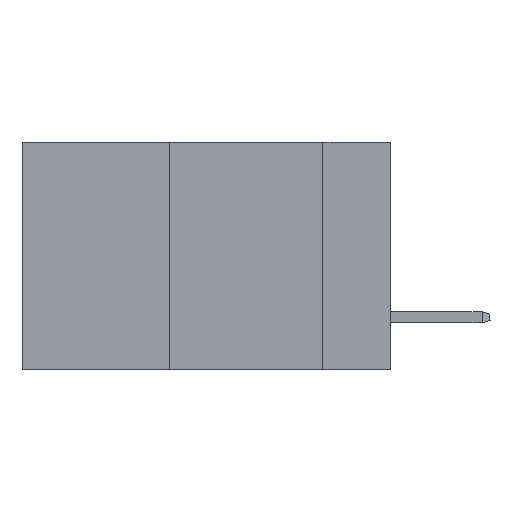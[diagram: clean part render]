
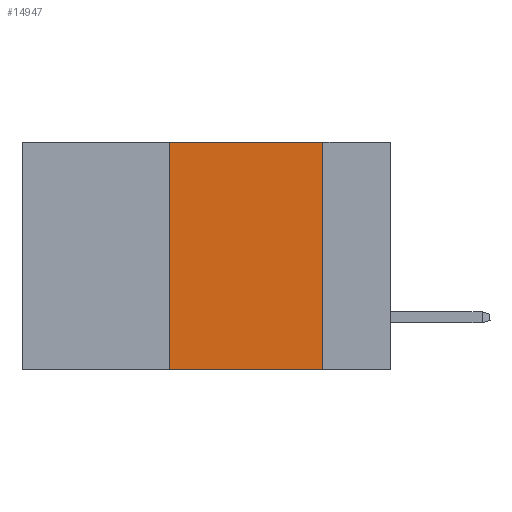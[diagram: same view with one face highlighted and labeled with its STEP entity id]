
A CAD part, left-side view. The second image highlights one B-rep face of the part: STEP entity #14947.
In plain terms, the highlighted planar face has unit normal (-1, 0, 0).
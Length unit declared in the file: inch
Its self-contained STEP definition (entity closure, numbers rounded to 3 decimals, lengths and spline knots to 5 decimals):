
#177 = VECTOR ( 'NONE', #9174, 39.37008 ) ;
#655 = VERTEX_POINT ( 'NONE', #10690 ) ;
#737 = CARTESIAN_POINT ( 'NONE',  ( 0., 0.6, 0. ) ) ;
#1632 = ORIENTED_EDGE ( 'NONE', *, *, #12199, .T. ) ;
#1851 = DIRECTION ( 'NONE',  ( 0., 0., -1. ) ) ;
#2074 = VECTOR ( 'NONE', #1851, 39.37008 ) ;
#2900 = CARTESIAN_POINT ( 'NONE',  ( 0., 0.36, 0. ) ) ;
#2974 = VECTOR ( 'NONE', #7356, 39.37008 ) ;
#4194 = LINE ( 'NONE', #6537, #2074 ) ;
#5190 = DIRECTION ( 'NONE',  ( 0., -1., 0. ) ) ;
#5197 = DIRECTION ( 'NONE',  ( 0., 0., -1. ) ) ;
#5221 = VECTOR ( 'NONE', #5190, 39.37008 ) ;
#5505 = VERTEX_POINT ( 'NONE', #14729 ) ;
#6537 = CARTESIAN_POINT ( 'NONE',  ( 0., 0.11, 0. ) ) ;
#6785 = EDGE_CURVE ( 'NONE', #16651, #11989, #14510, .T. ) ;
#7356 = DIRECTION ( 'NONE',  ( 0., -1., 0. ) ) ;
#8261 = CARTESIAN_POINT ( 'NONE',  ( 0., 0.36, -0.37 ) ) ;
#8672 = LINE ( 'NONE', #11134, #5221 ) ;
#9174 = DIRECTION ( 'NONE',  ( 0., 0., 1. ) ) ;
#9349 = LINE ( 'NONE', #14985, #2974 ) ;
#10690 = CARTESIAN_POINT ( 'NONE',  ( 0., 0.11, 0. ) ) ;
#11134 = CARTESIAN_POINT ( 'NONE',  ( 0., 0.6, -0.37 ) ) ;
#11989 = VERTEX_POINT ( 'NONE', #18265 ) ;
#12024 = EDGE_LOOP ( 'NONE', ( #18569, #13851, #15271, #1632 ) ) ;
#12199 = EDGE_CURVE ( 'NONE', #16651, #5505, #8672, .T. ) ;
#13851 = ORIENTED_EDGE ( 'NONE', *, *, #15005, .F. ) ;
#14143 = PLANE ( 'NONE',  #18775 ) ;
#14290 = EDGE_CURVE ( 'NONE', #655, #5505, #4194, .T. ) ;
#14510 = LINE ( 'NONE', #2900, #177 ) ;
#14729 = CARTESIAN_POINT ( 'NONE',  ( 0., 0.11, -0.37 ) ) ;
#14947 = ADVANCED_FACE ( 'NONE', ( #19365 ), #14143, .F. ) ;
#14985 = CARTESIAN_POINT ( 'NONE',  ( 0., 0.6, 0. ) ) ;
#15005 = EDGE_CURVE ( 'NONE', #11989, #655, #9349, .T. ) ;
#15271 = ORIENTED_EDGE ( 'NONE', *, *, #6785, .F. ) ;
#15726 = DIRECTION ( 'NONE',  ( 1., 0., 0. ) ) ;
#16651 = VERTEX_POINT ( 'NONE', #8261 ) ;
#18265 = CARTESIAN_POINT ( 'NONE',  ( 0., 0.36, 0. ) ) ;
#18569 = ORIENTED_EDGE ( 'NONE', *, *, #14290, .F. ) ;
#18775 = AXIS2_PLACEMENT_3D ( 'NONE', #737, #15726, #5197 ) ;
#19365 = FACE_OUTER_BOUND ( 'NONE', #12024, .T. ) ;
